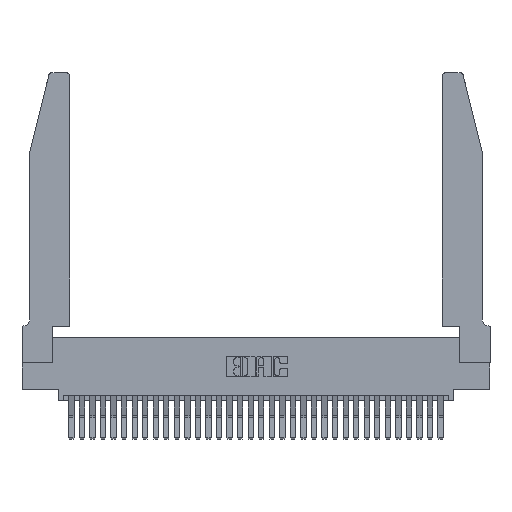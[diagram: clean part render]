
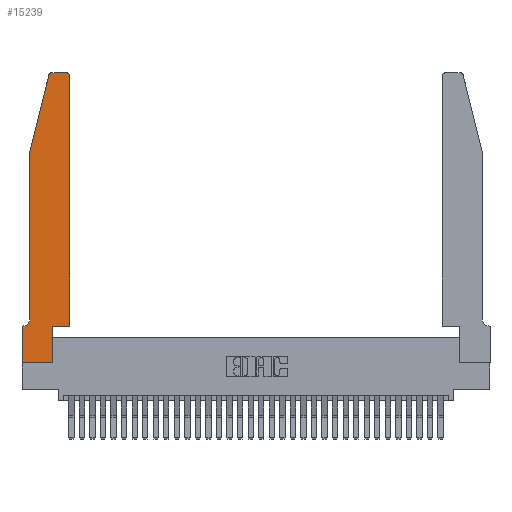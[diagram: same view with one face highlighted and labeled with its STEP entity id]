
A CAD part, top view. The second image highlights one B-rep face of the part: STEP entity #15239.
In plain terms, the highlighted planar face has unit normal (0, 0, 1).
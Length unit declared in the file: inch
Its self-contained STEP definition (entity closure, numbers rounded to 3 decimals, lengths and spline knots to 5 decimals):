
#112 = AXIS2_PLACEMENT_3D ( 'NONE', #14061, #32311, #16730 ) ;
#148 = CARTESIAN_POINT ( 'NONE',  ( 0.0055, 0.35, 0.37 ) ) ;
#402 = VERTEX_POINT ( 'NONE', #17119 ) ;
#992 = VERTEX_POINT ( 'NONE', #17082 ) ;
#1081 = LINE ( 'NONE', #30568, #27431 ) ;
#1123 = LINE ( 'NONE', #30411, #8206 ) ;
#1903 = VERTEX_POINT ( 'NONE', #26140 ) ;
#2263 = EDGE_LOOP ( 'NONE', ( #33940, #3855, #32344, #15231, #22891, #7146, #6722, #3358, #16008, #30624, #8369, #2574 ) ) ;
#2574 = ORIENTED_EDGE ( 'NONE', *, *, #21105, .T. ) ;
#2607 = CARTESIAN_POINT ( 'NONE',  ( 0.0755, 2., 0.37 ) ) ;
#2807 = LINE ( 'NONE', #2607, #29895 ) ;
#3358 = ORIENTED_EDGE ( 'NONE', *, *, #10874, .T. ) ;
#3855 = ORIENTED_EDGE ( 'NONE', *, *, #21455, .T. ) ;
#4273 = AXIS2_PLACEMENT_3D ( 'NONE', #5884, #8511, #26861 ) ;
#4287 = CIRCLE ( 'NONE', #33594, 0.03 ) ;
#4458 = CARTESIAN_POINT ( 'NONE',  ( 0.0755, 0.35, 0.37 ) ) ;
#4743 = DIRECTION ( 'NONE',  ( 0., -1., 0. ) ) ;
#5404 = CARTESIAN_POINT ( 'NONE',  ( 0.0055, 0.42, 0.37 ) ) ;
#5884 = CARTESIAN_POINT ( 'NONE',  ( 0., 0.35, 0.37 ) ) ;
#6266 = DIRECTION ( 'NONE',  ( -1., 0., 0. ) ) ;
#6722 = ORIENTED_EDGE ( 'NONE', *, *, #25667, .T. ) ;
#7135 = DIRECTION ( 'NONE',  ( -1., 0., 0. ) ) ;
#7146 = ORIENTED_EDGE ( 'NONE', *, *, #9913, .T. ) ;
#7291 = VERTEX_POINT ( 'NONE', #31178 ) ;
#7881 = DIRECTION ( 'NONE',  ( 0., 1., 0. ) ) ;
#8061 = DIRECTION ( 'NONE',  ( -1., 0., 0. ) ) ;
#8206 = VECTOR ( 'NONE', #33053, 39.37008 ) ;
#8369 = ORIENTED_EDGE ( 'NONE', *, *, #16332, .T. ) ;
#8511 = DIRECTION ( 'NONE',  ( 0., 0., 1. ) ) ;
#8928 = EDGE_CURVE ( 'NONE', #402, #7291, #24241, .T. ) ;
#9913 = EDGE_CURVE ( 'NONE', #19047, #33474, #17026, .T. ) ;
#9972 = VECTOR ( 'NONE', #7135, 39.37008 ) ;
#10215 = DIRECTION ( 'NONE',  ( 0., 0., 1. ) ) ;
#10465 = CIRCLE ( 'NONE', #17352, 0.07 ) ;
#10627 = VERTEX_POINT ( 'NONE', #15417 ) ;
#10874 = EDGE_CURVE ( 'NONE', #30701, #17739, #30361, .T. ) ;
#12202 = VECTOR ( 'NONE', #4743, 39.37008 ) ;
#12404 = EDGE_CURVE ( 'NONE', #17739, #13568, #1123, .T. ) ;
#12532 = CARTESIAN_POINT ( 'NONE',  ( 0., 0., 0.37 ) ) ;
#13568 = VERTEX_POINT ( 'NONE', #16942 ) ;
#13761 = CARTESIAN_POINT ( 'NONE',  ( 0., 0., 0.37 ) ) ;
#14061 = CARTESIAN_POINT ( 'NONE',  ( 0.4205, 2.72, 0.37 ) ) ;
#14097 = CARTESIAN_POINT ( 'NONE',  ( 0.4505, 0.35, 0.37 ) ) ;
#15128 = EDGE_CURVE ( 'NONE', #31451, #19047, #10465, .T. ) ;
#15231 = ORIENTED_EDGE ( 'NONE', *, *, #26371, .T. ) ;
#15239 = ADVANCED_FACE ( 'NONE', ( #27279 ), #24239, .T. ) ;
#15417 = CARTESIAN_POINT ( 'NONE',  ( 0.4505, 0.35, 0.37 ) ) ;
#16008 = ORIENTED_EDGE ( 'NONE', *, *, #12404, .T. ) ;
#16332 = EDGE_CURVE ( 'NONE', #10627, #1903, #20720, .T. ) ;
#16730 = DIRECTION ( 'NONE',  ( 1., 0., 0. ) ) ;
#16942 = CARTESIAN_POINT ( 'NONE',  ( 0.2865, 0.35, 0.37 ) ) ;
#17026 = LINE ( 'NONE', #4458, #9972 ) ;
#17082 = CARTESIAN_POINT ( 'NONE',  ( 0.25487, 2.72718, 0.37 ) ) ;
#17119 = CARTESIAN_POINT ( 'NONE',  ( 0.4205, 2.75, 0.37 ) ) ;
#17352 = AXIS2_PLACEMENT_3D ( 'NONE', #5404, #23800, #8061 ) ;
#17359 = VECTOR ( 'NONE', #21706, 39.37008 ) ;
#17739 = VERTEX_POINT ( 'NONE', #18977 ) ;
#18977 = CARTESIAN_POINT ( 'NONE',  ( 0.2865, 0., 0.37 ) ) ;
#19047 = VERTEX_POINT ( 'NONE', #148 ) ;
#19390 = DIRECTION ( 'NONE',  ( 1., 0., 0. ) ) ;
#19935 = LINE ( 'NONE', #14097, #32956 ) ;
#20720 = LINE ( 'NONE', #21025, #28421 ) ;
#21025 = CARTESIAN_POINT ( 'NONE',  ( 0.4505, 0.35, 0.37 ) ) ;
#21084 = DIRECTION ( 'NONE',  ( -0.239, -0.971, 0. ) ) ;
#21105 = EDGE_CURVE ( 'NONE', #1903, #402, #21242, .T. ) ;
#21242 = CIRCLE ( 'NONE', #112, 0.03 ) ;
#21455 = EDGE_CURVE ( 'NONE', #7291, #992, #4287, .T. ) ;
#21706 = DIRECTION ( 'NONE',  ( 1., 0., 0. ) ) ;
#22117 = CARTESIAN_POINT ( 'NONE',  ( 0.2605, 2.75, 0.37 ) ) ;
#22471 = EDGE_CURVE ( 'NONE', #13568, #10627, #19935, .T. ) ;
#22891 = ORIENTED_EDGE ( 'NONE', *, *, #15128, .T. ) ;
#22975 = CARTESIAN_POINT ( 'NONE',  ( 0.0755, 2., 0.37 ) ) ;
#23800 = DIRECTION ( 'NONE',  ( 0., 0., -1. ) ) ;
#24239 = PLANE ( 'NONE',  #4273 ) ;
#24241 = LINE ( 'NONE', #22117, #25886 ) ;
#25184 = EDGE_CURVE ( 'NONE', #992, #28308, #2807, .T. ) ;
#25561 = CARTESIAN_POINT ( 'NONE',  ( 0.0755, 2., 0.37 ) ) ;
#25667 = EDGE_CURVE ( 'NONE', #33474, #30701, #1081, .T. ) ;
#25886 = VECTOR ( 'NONE', #6266, 39.37008 ) ;
#25943 = CARTESIAN_POINT ( 'NONE',  ( 0.284, 2.72, 0.37 ) ) ;
#26140 = CARTESIAN_POINT ( 'NONE',  ( 0.4505, 2.72, 0.37 ) ) ;
#26371 = EDGE_CURVE ( 'NONE', #28308, #31451, #33915, .T. ) ;
#26861 = DIRECTION ( 'NONE',  ( 1., 0., 0. ) ) ;
#27279 = FACE_OUTER_BOUND ( 'NONE', #2263, .T. ) ;
#27431 = VECTOR ( 'NONE', #33220, 39.37008 ) ;
#28308 = VERTEX_POINT ( 'NONE', #22975 ) ;
#28421 = VECTOR ( 'NONE', #7881, 39.37008 ) ;
#28540 = DIRECTION ( 'NONE',  ( 1., 0., 0. ) ) ;
#29528 = CARTESIAN_POINT ( 'NONE',  ( 0., 0.35, 0.37 ) ) ;
#29895 = VECTOR ( 'NONE', #21084, 39.37008 ) ;
#30361 = LINE ( 'NONE', #13761, #17359 ) ;
#30411 = CARTESIAN_POINT ( 'NONE',  ( 0.2865, 0.35, 0.37 ) ) ;
#30568 = CARTESIAN_POINT ( 'NONE',  ( 0., 0., 0.37 ) ) ;
#30624 = ORIENTED_EDGE ( 'NONE', *, *, #22471, .T. ) ;
#30701 = VERTEX_POINT ( 'NONE', #12532 ) ;
#31013 = CARTESIAN_POINT ( 'NONE',  ( 0.0755, 0.42, 0.37 ) ) ;
#31178 = CARTESIAN_POINT ( 'NONE',  ( 0.284, 2.75, 0.37 ) ) ;
#31451 = VERTEX_POINT ( 'NONE', #31013 ) ;
#32311 = DIRECTION ( 'NONE',  ( 0., 0., 1. ) ) ;
#32344 = ORIENTED_EDGE ( 'NONE', *, *, #25184, .T. ) ;
#32956 = VECTOR ( 'NONE', #19390, 39.37008 ) ;
#33053 = DIRECTION ( 'NONE',  ( 0., 1., 0. ) ) ;
#33220 = DIRECTION ( 'NONE',  ( 0., -1., 0. ) ) ;
#33474 = VERTEX_POINT ( 'NONE', #29528 ) ;
#33594 = AXIS2_PLACEMENT_3D ( 'NONE', #25943, #10215, #28540 ) ;
#33915 = LINE ( 'NONE', #25561, #12202 ) ;
#33940 = ORIENTED_EDGE ( 'NONE', *, *, #8928, .T. ) ;
